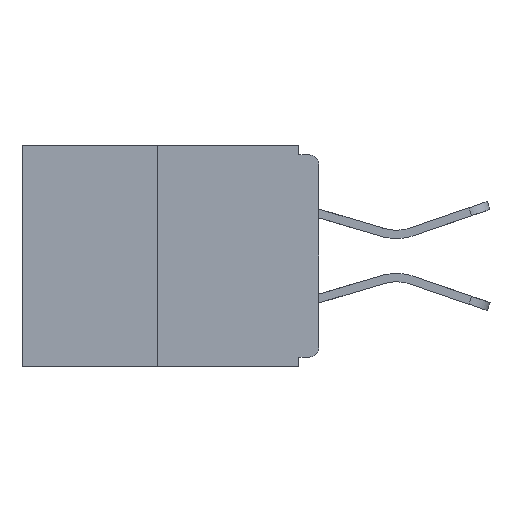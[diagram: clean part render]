
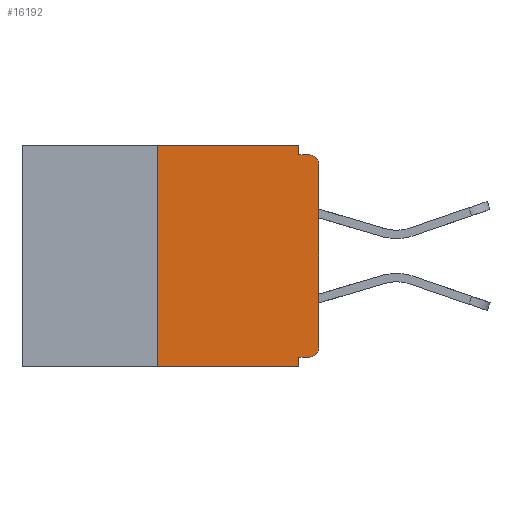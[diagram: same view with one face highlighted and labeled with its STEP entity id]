
A CAD part, left-side view. The second image highlights one B-rep face of the part: STEP entity #16192.
In plain terms, the highlighted planar face has unit normal (-1, 0, 0).
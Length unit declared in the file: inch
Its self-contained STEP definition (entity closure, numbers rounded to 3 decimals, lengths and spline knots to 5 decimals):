
#16 = CARTESIAN_POINT ( 'NONE',  ( 0., 0., -0.328 ) ) ;
#97 = PLANE ( 'NONE',  #8709 ) ;
#404 = CARTESIAN_POINT ( 'NONE',  ( 0., 0., -0.313 ) ) ;
#437 = ORIENTED_EDGE ( 'NONE', *, *, #9497, .F. ) ;
#582 = LINE ( 'NONE', #10220, #10758 ) ;
#585 = CARTESIAN_POINT ( 'NONE',  ( 0., 0.031, -0.343 ) ) ;
#970 = VECTOR ( 'NONE', #24554, 39.37008 ) ;
#1150 = EDGE_CURVE ( 'NONE', #21646, #8714, #582, .T. ) ;
#1732 = ORIENTED_EDGE ( 'NONE', *, *, #17146, .T. ) ;
#2000 = VERTEX_POINT ( 'NONE', #15535 ) ;
#2021 = EDGE_CURVE ( 'NONE', #17510, #2000, #17670, .T. ) ;
#2097 = ORIENTED_EDGE ( 'NONE', *, *, #4021, .F. ) ;
#2191 = CARTESIAN_POINT ( 'NONE',  ( 0., 0.25, 0. ) ) ;
#3440 = VERTEX_POINT ( 'NONE', #7778 ) ;
#3665 = EDGE_CURVE ( 'NONE', #2000, #3440, #23629, .T. ) ;
#3841 = ORIENTED_EDGE ( 'NONE', *, *, #3665, .T. ) ;
#4021 = EDGE_CURVE ( 'NONE', #8725, #21220, #13135, .T. ) ;
#4497 = DIRECTION ( 'NONE',  ( 0., 0., -1. ) ) ;
#4673 = EDGE_CURVE ( 'NONE', #9588, #18780, #22233, .T. ) ;
#5682 = AXIS2_PLACEMENT_3D ( 'NONE', #21942, #20195, #14303 ) ;
#5862 = CARTESIAN_POINT ( 'NONE',  ( 0., 0.031, -0.015 ) ) ;
#6242 = DIRECTION ( 'NONE',  ( 1., 0., 0. ) ) ;
#7740 = VECTOR ( 'NONE', #14354, 39.37008 ) ;
#7778 = CARTESIAN_POINT ( 'NONE',  ( 0., 0.015, -0.015 ) ) ;
#8167 = VECTOR ( 'NONE', #17650, 39.37008 ) ;
#8198 = FACE_OUTER_BOUND ( 'NONE', #9033, .T. ) ;
#8307 = DIRECTION ( 'NONE',  ( -1., 0., 0. ) ) ;
#8543 = ORIENTED_EDGE ( 'NONE', *, *, #17907, .T. ) ;
#8709 = AXIS2_PLACEMENT_3D ( 'NONE', #14336, #6242, #20410 ) ;
#8714 = VERTEX_POINT ( 'NONE', #5862 ) ;
#8725 = VERTEX_POINT ( 'NONE', #13753 ) ;
#9033 = EDGE_LOOP ( 'NONE', ( #21565, #10472, #1732, #14521, #2097, #8543, #24456, #3841, #437, #21431 ) ) ;
#9277 = CIRCLE ( 'NONE', #5682, 0.015 ) ;
#9426 = EDGE_CURVE ( 'NONE', #18780, #21646, #23880, .T. ) ;
#9497 = EDGE_CURVE ( 'NONE', #8714, #3440, #20993, .T. ) ;
#9588 = VERTEX_POINT ( 'NONE', #19586 ) ;
#10220 = CARTESIAN_POINT ( 'NONE',  ( 0., 0.031, 0. ) ) ;
#10472 = ORIENTED_EDGE ( 'NONE', *, *, #4673, .F. ) ;
#10758 = VECTOR ( 'NONE', #12067, 39.37008 ) ;
#10816 = CARTESIAN_POINT ( 'NONE',  ( 0., 0.46, -0.343 ) ) ;
#12052 = VECTOR ( 'NONE', #16998, 39.37008 ) ;
#12067 = DIRECTION ( 'NONE',  ( 0., 0., -1. ) ) ;
#13135 = LINE ( 'NONE', #16, #7740 ) ;
#13234 = CARTESIAN_POINT ( 'NONE',  ( 0., 0.46, 0. ) ) ;
#13633 = AXIS2_PLACEMENT_3D ( 'NONE', #24559, #8307, #4497 ) ;
#13753 = CARTESIAN_POINT ( 'NONE',  ( 0., 0.015, -0.328 ) ) ;
#13846 = CARTESIAN_POINT ( 'NONE',  ( 0., 0., -0.015 ) ) ;
#14303 = DIRECTION ( 'NONE',  ( 0., 0., -1. ) ) ;
#14317 = VECTOR ( 'NONE', #22720, 39.37008 ) ;
#14336 = CARTESIAN_POINT ( 'NONE',  ( 0., 0.46, 0. ) ) ;
#14354 = DIRECTION ( 'NONE',  ( 0., 1., 0. ) ) ;
#14521 = ORIENTED_EDGE ( 'NONE', *, *, #18834, .F. ) ;
#14694 = CARTESIAN_POINT ( 'NONE',  ( 0., 0.031, 0. ) ) ;
#14987 = CARTESIAN_POINT ( 'NONE',  ( 0., 0.25, 0. ) ) ;
#15476 = CARTESIAN_POINT ( 'NONE',  ( 0., 0.031, -0.343 ) ) ;
#15535 = CARTESIAN_POINT ( 'NONE',  ( 0., 0., -0.03 ) ) ;
#15792 = DIRECTION ( 'NONE',  ( 0., -1., 0. ) ) ;
#16192 = ADVANCED_FACE ( 'NONE', ( #8198 ), #97, .F. ) ;
#16998 = DIRECTION ( 'NONE',  ( 0., -1., 0. ) ) ;
#17144 = LINE ( 'NONE', #585, #970 ) ;
#17146 = EDGE_CURVE ( 'NONE', #9588, #23877, #21267, .T. ) ;
#17241 = CARTESIAN_POINT ( 'NONE',  ( 0., 0.031, -0.328 ) ) ;
#17281 = DIRECTION ( 'NONE',  ( 0., -1., 0. ) ) ;
#17510 = VERTEX_POINT ( 'NONE', #404 ) ;
#17650 = DIRECTION ( 'NONE',  ( 0., 0., 1. ) ) ;
#17670 = LINE ( 'NONE', #21848, #8167 ) ;
#17907 = EDGE_CURVE ( 'NONE', #8725, #17510, #9277, .T. ) ;
#18780 = VERTEX_POINT ( 'NONE', #2191 ) ;
#18834 = EDGE_CURVE ( 'NONE', #21220, #23877, #17144, .T. ) ;
#19586 = CARTESIAN_POINT ( 'NONE',  ( 0., 0.25, -0.343 ) ) ;
#20195 = DIRECTION ( 'NONE',  ( -1., 0., 0. ) ) ;
#20410 = DIRECTION ( 'NONE',  ( 0., 0., -1. ) ) ;
#20993 = LINE ( 'NONE', #13846, #24835 ) ;
#21220 = VERTEX_POINT ( 'NONE', #17241 ) ;
#21267 = LINE ( 'NONE', #10816, #12052 ) ;
#21431 = ORIENTED_EDGE ( 'NONE', *, *, #1150, .F. ) ;
#21565 = ORIENTED_EDGE ( 'NONE', *, *, #9426, .F. ) ;
#21646 = VERTEX_POINT ( 'NONE', #14694 ) ;
#21848 = CARTESIAN_POINT ( 'NONE',  ( 0., 0., 0. ) ) ;
#21942 = CARTESIAN_POINT ( 'NONE',  ( 0., 0.015, -0.313 ) ) ;
#22233 = LINE ( 'NONE', #14987, #14317 ) ;
#22720 = DIRECTION ( 'NONE',  ( 0., 0., 1. ) ) ;
#23245 = VECTOR ( 'NONE', #17281, 39.37008 ) ;
#23629 = CIRCLE ( 'NONE', #13633, 0.015 ) ;
#23877 = VERTEX_POINT ( 'NONE', #15476 ) ;
#23880 = LINE ( 'NONE', #13234, #23245 ) ;
#24456 = ORIENTED_EDGE ( 'NONE', *, *, #2021, .T. ) ;
#24554 = DIRECTION ( 'NONE',  ( 0., 0., -1. ) ) ;
#24559 = CARTESIAN_POINT ( 'NONE',  ( 0., 0.015, -0.03 ) ) ;
#24835 = VECTOR ( 'NONE', #15792, 39.37008 ) ;
